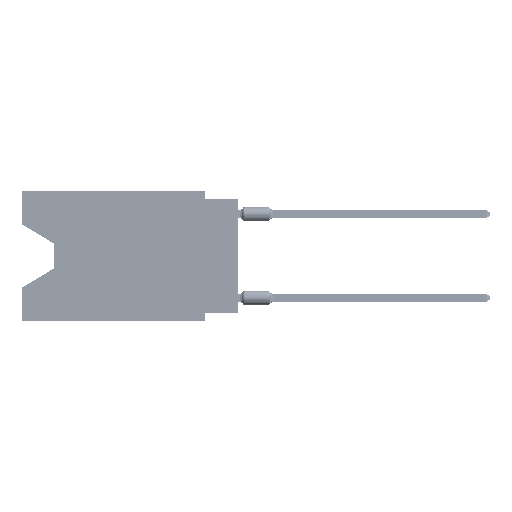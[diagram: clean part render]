
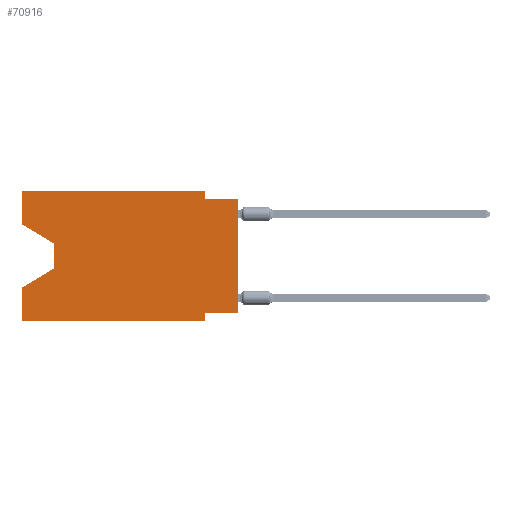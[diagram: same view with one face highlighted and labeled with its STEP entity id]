
A CAD part, left-side view. The second image highlights one B-rep face of the part: STEP entity #70916.
In plain terms, the highlighted planar face has unit normal (-1, 0, 0).
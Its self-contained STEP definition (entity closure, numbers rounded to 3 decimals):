
#1591 = EDGE_CURVE ( 'NONE', #3837, #66687, #63586, .T. ) ;
#2212 = CARTESIAN_POINT ( 'NONE',  ( 0., 2.54, 0. ) ) ;
#2990 = CARTESIAN_POINT ( 'NONE',  ( 0., 16.383, 0. ) ) ;
#3837 = VERTEX_POINT ( 'NONE', #19364 ) ;
#5411 = CARTESIAN_POINT ( 'NONE',  ( 0., 2.54, -9.271 ) ) ;
#5650 = LINE ( 'NONE', #22710, #33510 ) ;
#6369 = CARTESIAN_POINT ( 'NONE',  ( 0., 16.383, 0. ) ) ;
#6939 = VECTOR ( 'NONE', #47333, 1000. ) ;
#7025 = EDGE_CURVE ( 'NONE', #25725, #60495, #62939, .T. ) ;
#7105 = CARTESIAN_POINT ( 'NONE',  ( 0., 0., -0.635 ) ) ;
#8755 = VECTOR ( 'NONE', #22298, 1000. ) ;
#8908 = DIRECTION ( 'NONE',  ( 0., 0., 1. ) ) ;
#10994 = VERTEX_POINT ( 'NONE', #63744 ) ;
#14194 = EDGE_CURVE ( 'NONE', #60841, #35650, #63223, .T. ) ;
#14363 = DIRECTION ( 'NONE',  ( 0., 0., 1. ) ) ;
#15299 = ORIENTED_EDGE ( 'NONE', *, *, #33698, .F. ) ;
#15481 = EDGE_LOOP ( 'NONE', ( #48715, #41732, #37069, #42327, #53119, #20565, #58510, #57864, #15299, #47967, #54467, #22011 ) ) ;
#16561 = VECTOR ( 'NONE', #51905, 1000. ) ;
#17149 = VECTOR ( 'NONE', #66993, 1000. ) ;
#17893 = VECTOR ( 'NONE', #47575, 1000. ) ;
#18021 = CARTESIAN_POINT ( 'NONE',  ( 0., 16.383, -9.906 ) ) ;
#18178 = VECTOR ( 'NONE', #8908, 1000. ) ;
#19113 = DIRECTION ( 'NONE',  ( 0., -1., 0. ) ) ;
#19364 = CARTESIAN_POINT ( 'NONE',  ( 0., 16.383, -9.906 ) ) ;
#20565 = ORIENTED_EDGE ( 'NONE', *, *, #45322, .F. ) ;
#20654 = EDGE_CURVE ( 'NONE', #60495, #27936, #68190, .T. ) ;
#21792 = CARTESIAN_POINT ( 'NONE',  ( 0., 16.383, 0. ) ) ;
#22011 = ORIENTED_EDGE ( 'NONE', *, *, #45590, .F. ) ;
#22094 = CARTESIAN_POINT ( 'NONE',  ( 0., 13.97, -4.013 ) ) ;
#22298 = DIRECTION ( 'NONE',  ( 0., 0.855, -0.519 ) ) ;
#22710 = CARTESIAN_POINT ( 'NONE',  ( 0., 2.54, -9.906 ) ) ;
#25725 = VERTEX_POINT ( 'NONE', #41985 ) ;
#25873 = CARTESIAN_POINT ( 'NONE',  ( 0., 2.54, -9.906 ) ) ;
#26206 = VERTEX_POINT ( 'NONE', #7105 ) ;
#27798 = CARTESIAN_POINT ( 'NONE',  ( 0., 2.54, 0. ) ) ;
#27835 = VERTEX_POINT ( 'NONE', #42952 ) ;
#27852 = PLANE ( 'NONE',  #37566 ) ;
#27936 = VERTEX_POINT ( 'NONE', #72581 ) ;
#28491 = VERTEX_POINT ( 'NONE', #5411 ) ;
#31244 = LINE ( 'NONE', #71616, #17893 ) ;
#31355 = LINE ( 'NONE', #64369, #6939 ) ;
#33510 = VECTOR ( 'NONE', #45316, 1000. ) ;
#33698 = EDGE_CURVE ( 'NONE', #27936, #26206, #72904, .T. ) ;
#34099 = VECTOR ( 'NONE', #14363, 1000. ) ;
#34709 = DIRECTION ( 'NONE',  ( 0., 0., -1. ) ) ;
#35650 = VERTEX_POINT ( 'NONE', #60061 ) ;
#35947 = EDGE_CURVE ( 'NONE', #10994, #28491, #31355, .T. ) ;
#37069 = ORIENTED_EDGE ( 'NONE', *, *, #64992, .T. ) ;
#37566 = AXIS2_PLACEMENT_3D ( 'NONE', #6369, #46030, #67534 ) ;
#41732 = ORIENTED_EDGE ( 'NONE', *, *, #14194, .T. ) ;
#41985 = CARTESIAN_POINT ( 'NONE',  ( 0., 16.383, 0. ) ) ;
#42327 = ORIENTED_EDGE ( 'NONE', *, *, #49094, .F. ) ;
#42952 = CARTESIAN_POINT ( 'NONE',  ( 0., 16.383, -7.36 ) ) ;
#43247 = LINE ( 'NONE', #65146, #34099 ) ;
#43916 = EDGE_CURVE ( 'NONE', #62028, #60841, #31244, .T. ) ;
#45316 = DIRECTION ( 'NONE',  ( 0., 0., -1. ) ) ;
#45322 = EDGE_CURVE ( 'NONE', #28491, #66687, #5650, .T. ) ;
#45590 = EDGE_CURVE ( 'NONE', #62028, #25725, #60449, .T. ) ;
#46030 = DIRECTION ( 'NONE',  ( 1., 0., 0. ) ) ;
#47333 = DIRECTION ( 'NONE',  ( 0., 1., 0. ) ) ;
#47575 = DIRECTION ( 'NONE',  ( 0., -0.855, -0.519 ) ) ;
#47967 = ORIENTED_EDGE ( 'NONE', *, *, #20654, .F. ) ;
#48715 = ORIENTED_EDGE ( 'NONE', *, *, #43916, .T. ) ;
#48953 = CARTESIAN_POINT ( 'NONE',  ( 0., 16.383, -2.546 ) ) ;
#49094 = EDGE_CURVE ( 'NONE', #3837, #27835, #56255, .T. ) ;
#49815 = VECTOR ( 'NONE', #66988, 1000. ) ;
#51422 = CARTESIAN_POINT ( 'NONE',  ( 0., 0., -0.635 ) ) ;
#51854 = VECTOR ( 'NONE', #19113, 1000. ) ;
#51905 = DIRECTION ( 'NONE',  ( 0., 0., -1. ) ) ;
#53119 = ORIENTED_EDGE ( 'NONE', *, *, #1591, .T. ) ;
#54467 = ORIENTED_EDGE ( 'NONE', *, *, #7025, .F. ) ;
#55279 = LINE ( 'NONE', #61944, #8755 ) ;
#55541 = CARTESIAN_POINT ( 'NONE',  ( 0., 16.383, 0. ) ) ;
#56255 = LINE ( 'NONE', #55541, #17149 ) ;
#57792 = VECTOR ( 'NONE', #62162, 1000. ) ;
#57864 = ORIENTED_EDGE ( 'NONE', *, *, #69893, .T. ) ;
#58510 = ORIENTED_EDGE ( 'NONE', *, *, #35947, .F. ) ;
#60061 = CARTESIAN_POINT ( 'NONE',  ( 0., 13.97, -5.893 ) ) ;
#60449 = LINE ( 'NONE', #2990, #18178 ) ;
#60495 = VERTEX_POINT ( 'NONE', #27798 ) ;
#60841 = VERTEX_POINT ( 'NONE', #72564 ) ;
#61944 = CARTESIAN_POINT ( 'NONE',  ( 0., 13.97, -5.893 ) ) ;
#62028 = VERTEX_POINT ( 'NONE', #48953 ) ;
#62162 = DIRECTION ( 'NONE',  ( 0., -1., 0. ) ) ;
#62939 = LINE ( 'NONE', #21792, #49815 ) ;
#63223 = LINE ( 'NONE', #22094, #63626 ) ;
#63586 = LINE ( 'NONE', #18021, #51854 ) ;
#63626 = VECTOR ( 'NONE', #34709, 1000. ) ;
#63744 = CARTESIAN_POINT ( 'NONE',  ( 0., 0., -9.271 ) ) ;
#64369 = CARTESIAN_POINT ( 'NONE',  ( 0., 0., -9.271 ) ) ;
#64992 = EDGE_CURVE ( 'NONE', #35650, #27835, #55279, .T. ) ;
#65146 = CARTESIAN_POINT ( 'NONE',  ( 0., 0., 0. ) ) ;
#66687 = VERTEX_POINT ( 'NONE', #25873 ) ;
#66988 = DIRECTION ( 'NONE',  ( 0., -1., 0. ) ) ;
#66993 = DIRECTION ( 'NONE',  ( 0., 0., 1. ) ) ;
#67534 = DIRECTION ( 'NONE',  ( 0., 0., -1. ) ) ;
#67890 = FACE_OUTER_BOUND ( 'NONE', #15481, .T. ) ;
#68190 = LINE ( 'NONE', #2212, #16561 ) ;
#69893 = EDGE_CURVE ( 'NONE', #10994, #26206, #43247, .T. ) ;
#70916 = ADVANCED_FACE ( 'NONE', ( #67890 ), #27852, .F. ) ;
#71616 = CARTESIAN_POINT ( 'NONE',  ( 0., 16.383, -2.546 ) ) ;
#72564 = CARTESIAN_POINT ( 'NONE',  ( 0., 13.97, -4.013 ) ) ;
#72581 = CARTESIAN_POINT ( 'NONE',  ( 0., 2.54, -0.635 ) ) ;
#72904 = LINE ( 'NONE', #51422, #57792 ) ;
